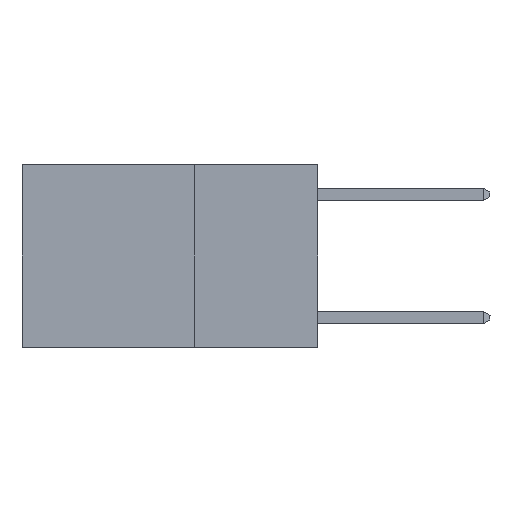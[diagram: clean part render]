
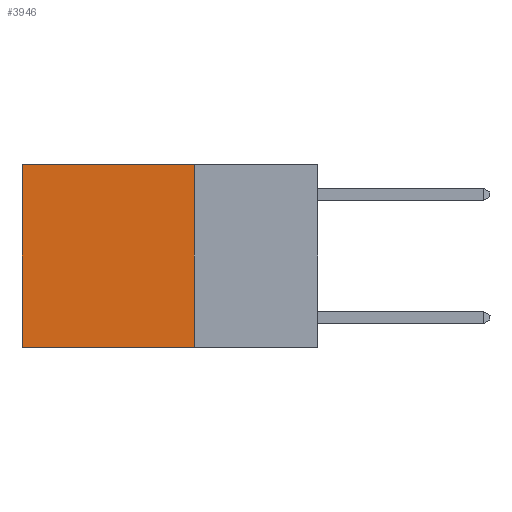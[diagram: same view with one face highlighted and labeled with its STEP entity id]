
A CAD part, left-side view. The second image highlights one B-rep face of the part: STEP entity #3946.
In plain terms, the highlighted planar face has unit normal (-1, 0, 0).
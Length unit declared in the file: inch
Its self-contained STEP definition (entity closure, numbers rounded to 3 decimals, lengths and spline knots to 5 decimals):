
#2647 = AXIS2_PLACEMENT_3D ( 'NONE', #23845, #25929, #13176 ) ;
#3260 = VERTEX_POINT ( 'NONE', #5017 ) ;
#3946 = ADVANCED_FACE ( 'NONE', ( #21675 ), #8662, .F. ) ;
#4655 = DIRECTION ( 'NONE',  ( 0., 1., 0. ) ) ;
#4882 = ORIENTED_EDGE ( 'NONE', *, *, #20280, .T. ) ;
#5017 = CARTESIAN_POINT ( 'NONE',  ( 0.2625, 0.6, -0.37 ) ) ;
#5088 = ORIENTED_EDGE ( 'NONE', *, *, #11286, .F. ) ;
#5369 = LINE ( 'NONE', #13819, #10853 ) ;
#5631 = ORIENTED_EDGE ( 'NONE', *, *, #20745, .F. ) ;
#5868 = VECTOR ( 'NONE', #13794, 39.37008 ) ;
#6067 = CARTESIAN_POINT ( 'NONE',  ( 0.2625, 0.25, -0.37 ) ) ;
#6143 = ORIENTED_EDGE ( 'NONE', *, *, #22069, .T. ) ;
#6353 = VERTEX_POINT ( 'NONE', #23487 ) ;
#7069 = CARTESIAN_POINT ( 'NONE',  ( 0.2625, 0.6, 0. ) ) ;
#8662 = PLANE ( 'NONE',  #2647 ) ;
#10853 = VECTOR ( 'NONE', #4655, 39.37008 ) ;
#11286 = EDGE_CURVE ( 'NONE', #20879, #3260, #26056, .T. ) ;
#12612 = VECTOR ( 'NONE', #19273, 39.37008 ) ;
#12730 = CARTESIAN_POINT ( 'NONE',  ( 0.2625, 0.25, 0. ) ) ;
#13176 = DIRECTION ( 'NONE',  ( 0., 0., -1. ) ) ;
#13794 = DIRECTION ( 'NONE',  ( 0., 0., -1. ) ) ;
#13819 = CARTESIAN_POINT ( 'NONE',  ( 0.2625, 0.25, 0. ) ) ;
#13973 = LINE ( 'NONE', #12730, #12612 ) ;
#14142 = CARTESIAN_POINT ( 'NONE',  ( 0.2625, 0.25, -0.37 ) ) ;
#14829 = EDGE_LOOP ( 'NONE', ( #4882, #5088, #5631, #6143 ) ) ;
#17745 = LINE ( 'NONE', #7069, #5868 ) ;
#18942 = CARTESIAN_POINT ( 'NONE',  ( 0.2625, 0.6, 0. ) ) ;
#19273 = DIRECTION ( 'NONE',  ( 0., 0., -1. ) ) ;
#19728 = VERTEX_POINT ( 'NONE', #18942 ) ;
#19821 = VECTOR ( 'NONE', #24948, 39.37008 ) ;
#20280 = EDGE_CURVE ( 'NONE', #19728, #3260, #17745, .T. ) ;
#20745 = EDGE_CURVE ( 'NONE', #6353, #20879, #13973, .T. ) ;
#20879 = VERTEX_POINT ( 'NONE', #6067 ) ;
#21675 = FACE_OUTER_BOUND ( 'NONE', #14829, .T. ) ;
#22069 = EDGE_CURVE ( 'NONE', #6353, #19728, #5369, .T. ) ;
#23487 = CARTESIAN_POINT ( 'NONE',  ( 0.2625, 0.25, 0. ) ) ;
#23845 = CARTESIAN_POINT ( 'NONE',  ( 0.2625, 0.25, 0. ) ) ;
#24948 = DIRECTION ( 'NONE',  ( 0., 1., 0. ) ) ;
#25929 = DIRECTION ( 'NONE',  ( 1., 0., 0. ) ) ;
#26056 = LINE ( 'NONE', #14142, #19821 ) ;
